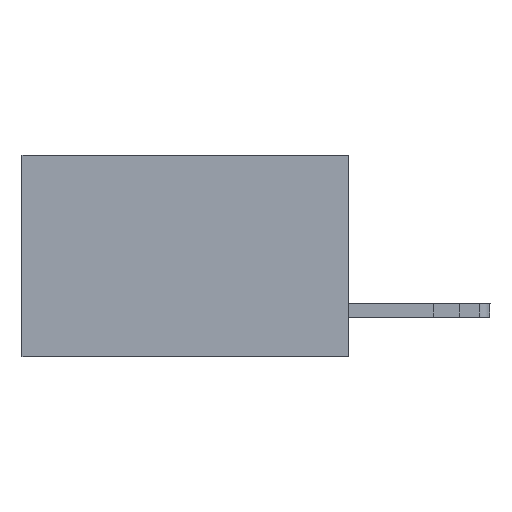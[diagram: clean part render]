
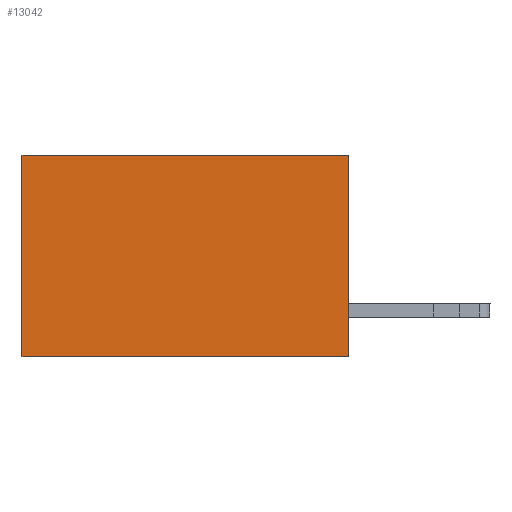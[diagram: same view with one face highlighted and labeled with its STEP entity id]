
A CAD part, left-side view. The second image highlights one B-rep face of the part: STEP entity #13042.
In plain terms, the highlighted planar face has unit normal (-1, 0, 0).
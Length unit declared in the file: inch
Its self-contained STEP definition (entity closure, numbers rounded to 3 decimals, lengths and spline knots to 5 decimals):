
#857 = VECTOR ( 'NONE', #13446, 39.37008 ) ;
#1017 = DIRECTION ( 'NONE',  ( 1., 0., 0. ) ) ;
#1236 = VECTOR ( 'NONE', #10291, 39.37008 ) ;
#1253 = DIRECTION ( 'NONE',  ( 0., 0., -1. ) ) ;
#2151 = DIRECTION ( 'NONE',  ( 0., 0., -1. ) ) ;
#2684 = ORIENTED_EDGE ( 'NONE', *, *, #6855, .F. ) ;
#2921 = VERTEX_POINT ( 'NONE', #9463 ) ;
#2982 = VERTEX_POINT ( 'NONE', #8317 ) ;
#3692 = DIRECTION ( 'NONE',  ( 0., 1., 0. ) ) ;
#4041 = ORIENTED_EDGE ( 'NONE', *, *, #10617, .T. ) ;
#4052 = CARTESIAN_POINT ( 'NONE',  ( 0.298, 0., 0. ) ) ;
#4187 = CARTESIAN_POINT ( 'NONE',  ( 0.298, 0., 0. ) ) ;
#4204 = LINE ( 'NONE', #6885, #1236 ) ;
#4314 = AXIS2_PLACEMENT_3D ( 'NONE', #4187, #1017, #2151 ) ;
#5749 = CARTESIAN_POINT ( 'NONE',  ( 0.298, 0.6, 0. ) ) ;
#6511 = EDGE_CURVE ( 'NONE', #13808, #2982, #11164, .T. ) ;
#6561 = EDGE_LOOP ( 'NONE', ( #7172, #11977, #2684, #4041 ) ) ;
#6647 = VECTOR ( 'NONE', #3692, 39.37008 ) ;
#6831 = FACE_OUTER_BOUND ( 'NONE', #6561, .T. ) ;
#6855 = EDGE_CURVE ( 'NONE', #10317, #2921, #7037, .T. ) ;
#6885 = CARTESIAN_POINT ( 'NONE',  ( 0.298, 0., 0. ) ) ;
#7037 = LINE ( 'NONE', #7922, #14305 ) ;
#7172 = ORIENTED_EDGE ( 'NONE', *, *, #6511, .T. ) ;
#7655 = CARTESIAN_POINT ( 'NONE',  ( 0.298, 0.6, 0. ) ) ;
#7922 = CARTESIAN_POINT ( 'NONE',  ( 0.298, 0., 0. ) ) ;
#8317 = CARTESIAN_POINT ( 'NONE',  ( 0.298, 0.6, -0.37 ) ) ;
#8699 = PLANE ( 'NONE',  #4314 ) ;
#8817 = EDGE_CURVE ( 'NONE', #2921, #2982, #10931, .T. ) ;
#9155 = CARTESIAN_POINT ( 'NONE',  ( 0.298, 0., -0.37 ) ) ;
#9463 = CARTESIAN_POINT ( 'NONE',  ( 0.298, 0., -0.37 ) ) ;
#10291 = DIRECTION ( 'NONE',  ( 0., 1., 0. ) ) ;
#10317 = VERTEX_POINT ( 'NONE', #4052 ) ;
#10617 = EDGE_CURVE ( 'NONE', #10317, #13808, #4204, .T. ) ;
#10931 = LINE ( 'NONE', #9155, #6647 ) ;
#11164 = LINE ( 'NONE', #5749, #857 ) ;
#11977 = ORIENTED_EDGE ( 'NONE', *, *, #8817, .F. ) ;
#13042 = ADVANCED_FACE ( 'NONE', ( #6831 ), #8699, .F. ) ;
#13446 = DIRECTION ( 'NONE',  ( 0., 0., -1. ) ) ;
#13808 = VERTEX_POINT ( 'NONE', #7655 ) ;
#14305 = VECTOR ( 'NONE', #1253, 39.37008 ) ;
